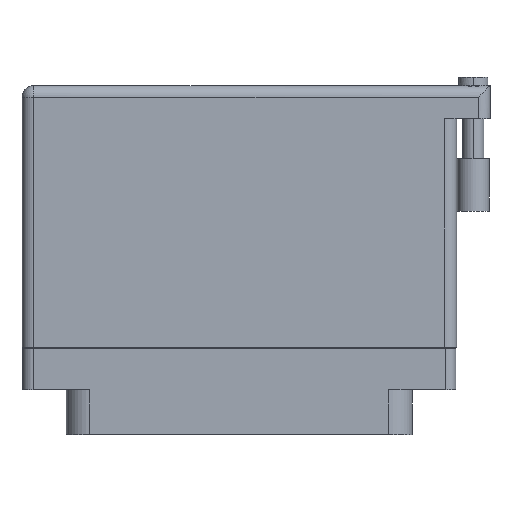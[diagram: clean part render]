
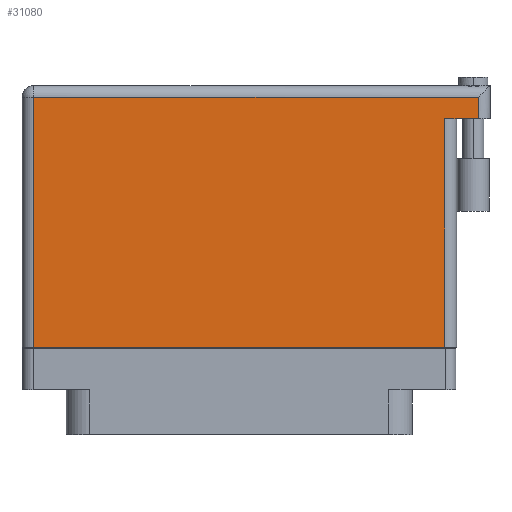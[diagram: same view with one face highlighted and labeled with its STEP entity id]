
A CAD part, front view. The second image highlights one B-rep face of the part: STEP entity #31080.
In plain terms, the highlighted face is planar.
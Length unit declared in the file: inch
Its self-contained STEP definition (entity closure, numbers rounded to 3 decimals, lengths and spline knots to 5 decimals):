
#1242 = VECTOR ( 'NONE', #29466, 39.37008 ) ;
#1793 = VECTOR ( 'NONE', #42877, 39.37008 ) ;
#2193 = EDGE_CURVE ( 'NONE', #35185, #45120, #30481, .T. ) ;
#3564 = CARTESIAN_POINT ( 'NONE',  ( 1.43, 1.269, 0.4495 ) ) ;
#3786 = DIRECTION ( 'NONE',  ( 0., -1., 0. ) ) ;
#5832 = CARTESIAN_POINT ( 'NONE',  ( 1.23, 1.269, 0.4495 ) ) ;
#7801 = AXIS2_PLACEMENT_3D ( 'NONE', #46813, #51393, #11624 ) ;
#9333 = VECTOR ( 'NONE', #27365, 39.37008 ) ;
#11624 = DIRECTION ( 'NONE',  ( -1., 0., 0. ) ) ;
#12385 = ORIENTED_EDGE ( 'NONE', *, *, #14740, .T. ) ;
#14389 = LINE ( 'NONE', #33751, #28095 ) ;
#14740 = EDGE_CURVE ( 'NONE', #37217, #45120, #48605, .T. ) ;
#15007 = CARTESIAN_POINT ( 'NONE',  ( 1.5, 1.269, 0.4495 ) ) ;
#18233 = CARTESIAN_POINT ( 'NONE',  ( 1.43, 1.396, 0.4495 ) ) ;
#18462 = LINE ( 'NONE', #37073, #48871 ) ;
#18474 = DIRECTION ( 'NONE',  ( -1., 0., 0. ) ) ;
#18505 = CARTESIAN_POINT ( 'NONE',  ( 1.23, -0.1, 0.4495 ) ) ;
#19031 = PLANE ( 'NONE',  #7801 ) ;
#19315 = CARTESIAN_POINT ( 'NONE',  ( -1.23, 1.396, 0.4495 ) ) ;
#20705 = ORIENTED_EDGE ( 'NONE', *, *, #29105, .T. ) ;
#22726 = CARTESIAN_POINT ( 'NONE',  ( 1.43, 1.466, 0.4495 ) ) ;
#23015 = LINE ( 'NONE', #22726, #1793 ) ;
#24293 = FACE_OUTER_BOUND ( 'NONE', #44596, .T. ) ;
#25115 = ORIENTED_EDGE ( 'NONE', *, *, #25135, .T. ) ;
#25135 = EDGE_CURVE ( 'NONE', #26878, #41384, #14389, .T. ) ;
#25832 = LINE ( 'NONE', #47652, #33898 ) ;
#26878 = VERTEX_POINT ( 'NONE', #18233 ) ;
#27365 = DIRECTION ( 'NONE',  ( -1., 0., 0. ) ) ;
#28095 = VECTOR ( 'NONE', #18474, 39.37008 ) ;
#28751 = EDGE_CURVE ( 'NONE', #36696, #37217, #18462, .T. ) ;
#29105 = EDGE_CURVE ( 'NONE', #41384, #36696, #25832, .T. ) ;
#29466 = DIRECTION ( 'NONE',  ( 0., 1., 0. ) ) ;
#30481 = LINE ( 'NONE', #15007, #9333 ) ;
#31080 = ADVANCED_FACE ( 'NONE', ( #24293 ), #19031, .F. ) ;
#31372 = CARTESIAN_POINT ( 'NONE',  ( 1.23, 1.269, 0.4495 ) ) ;
#32764 = DIRECTION ( 'NONE',  ( 1., 0., 0. ) ) ;
#32994 = CARTESIAN_POINT ( 'NONE',  ( -1.23, -0.1, 0.4495 ) ) ;
#33751 = CARTESIAN_POINT ( 'NONE',  ( -1.3, 1.396, 0.4495 ) ) ;
#33898 = VECTOR ( 'NONE', #3786, 39.37008 ) ;
#35185 = VERTEX_POINT ( 'NONE', #3564 ) ;
#35187 = ORIENTED_EDGE ( 'NONE', *, *, #28751, .T. ) ;
#36696 = VERTEX_POINT ( 'NONE', #32994 ) ;
#37073 = CARTESIAN_POINT ( 'NONE',  ( -1.3, -0.1, 0.4495 ) ) ;
#37217 = VERTEX_POINT ( 'NONE', #18505 ) ;
#38606 = ORIENTED_EDGE ( 'NONE', *, *, #45010, .T. ) ;
#38999 = ORIENTED_EDGE ( 'NONE', *, *, #2193, .F. ) ;
#41384 = VERTEX_POINT ( 'NONE', #19315 ) ;
#42877 = DIRECTION ( 'NONE',  ( 0., 1., 0. ) ) ;
#44596 = EDGE_LOOP ( 'NONE', ( #35187, #12385, #38999, #38606, #25115, #20705 ) ) ;
#45010 = EDGE_CURVE ( 'NONE', #35185, #26878, #23015, .T. ) ;
#45120 = VERTEX_POINT ( 'NONE', #31372 ) ;
#46813 = CARTESIAN_POINT ( 'NONE',  ( -1.3, 1.466, 0.4495 ) ) ;
#47652 = CARTESIAN_POINT ( 'NONE',  ( -1.23, -0.1, 0.4495 ) ) ;
#48605 = LINE ( 'NONE', #5832, #1242 ) ;
#48871 = VECTOR ( 'NONE', #32764, 39.37008 ) ;
#51393 = DIRECTION ( 'NONE',  ( 0., 0., -1. ) ) ;
